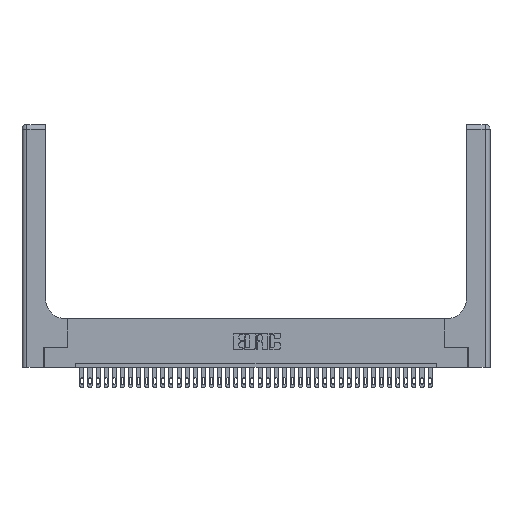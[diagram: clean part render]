
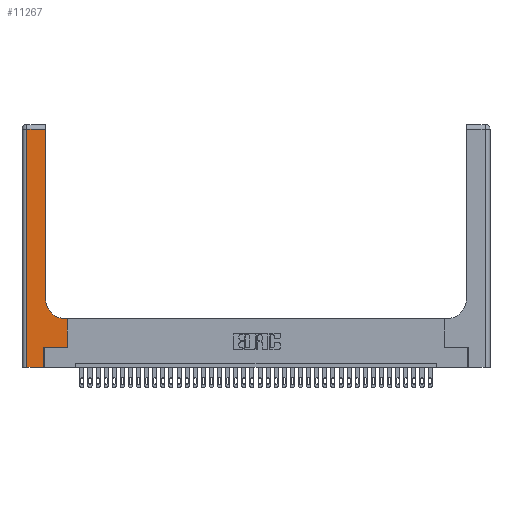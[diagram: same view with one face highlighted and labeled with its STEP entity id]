
A CAD part, top view. The second image highlights one B-rep face of the part: STEP entity #11267.
In plain terms, the highlighted planar face has unit normal (0, 0, 1).
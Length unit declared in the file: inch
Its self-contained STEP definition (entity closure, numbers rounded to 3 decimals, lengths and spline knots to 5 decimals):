
#680 = CARTESIAN_POINT ( 'NONE',  ( 0.06, 0., 0.37 ) ) ;
#816 = EDGE_CURVE ( 'NONE', #2927, #21546, #34071, .T. ) ;
#1588 = DIRECTION ( 'NONE',  ( 1., 0., 0. ) ) ;
#2129 = CARTESIAN_POINT ( 'NONE',  ( 0.2915, 3., 0.37 ) ) ;
#2460 = ORIENTED_EDGE ( 'NONE', *, *, #816, .T. ) ;
#2927 = VERTEX_POINT ( 'NONE', #27024 ) ;
#3459 = VECTOR ( 'NONE', #21099, 39.37008 ) ;
#3595 = ORIENTED_EDGE ( 'NONE', *, *, #24261, .T. ) ;
#3907 = CARTESIAN_POINT ( 'NONE',  ( 0.5585, 0.25, 0.37 ) ) ;
#4090 = ORIENTED_EDGE ( 'NONE', *, *, #33773, .T. ) ;
#4629 = VECTOR ( 'NONE', #26084, 39.37008 ) ;
#4866 = VERTEX_POINT ( 'NONE', #36740 ) ;
#4934 = DIRECTION ( 'NONE',  ( 1., 0., 0. ) ) ;
#5046 = EDGE_CURVE ( 'NONE', #28996, #8371, #12934, .T. ) ;
#5587 = DIRECTION ( 'NONE',  ( 0., 1., 0. ) ) ;
#5612 = PLANE ( 'NONE',  #34183 ) ;
#6397 = VECTOR ( 'NONE', #1588, 39.37008 ) ;
#6683 = EDGE_CURVE ( 'NONE', #35294, #28996, #28286, .T. ) ;
#8371 = VERTEX_POINT ( 'NONE', #13089 ) ;
#8490 = CARTESIAN_POINT ( 'NONE',  ( 0.5415, 0.6, 0.37 ) ) ;
#9694 = LINE ( 'NONE', #10641, #28366 ) ;
#9822 = ORIENTED_EDGE ( 'NONE', *, *, #26057, .T. ) ;
#10203 = VECTOR ( 'NONE', #5587, 39.37008 ) ;
#10488 = ORIENTED_EDGE ( 'NONE', *, *, #5046, .T. ) ;
#10577 = LINE ( 'NONE', #34936, #4629 ) ;
#10641 = CARTESIAN_POINT ( 'NONE',  ( 0.06, 3., 0.37 ) ) ;
#11267 = ADVANCED_FACE ( 'NONE', ( #24616 ), #5612, .F. ) ;
#11600 = ORIENTED_EDGE ( 'NONE', *, *, #12400, .T. ) ;
#11877 = ORIENTED_EDGE ( 'NONE', *, *, #37882, .T. ) ;
#11999 = CARTESIAN_POINT ( 'NONE',  ( 0.5585, 0.25, 0.37 ) ) ;
#12116 = CARTESIAN_POINT ( 'NONE',  ( 0.269, 0.25, 0.37 ) ) ;
#12400 = EDGE_CURVE ( 'NONE', #21546, #4866, #32258, .T. ) ;
#12431 = CIRCLE ( 'NONE', #13521, 0.25 ) ;
#12934 = LINE ( 'NONE', #3907, #10203 ) ;
#13089 = CARTESIAN_POINT ( 'NONE',  ( 0.5585, 0.6, 0.37 ) ) ;
#13521 = AXIS2_PLACEMENT_3D ( 'NONE', #31881, #22835, #16991 ) ;
#13764 = VECTOR ( 'NONE', #4934, 39.37008 ) ;
#16405 = CARTESIAN_POINT ( 'NONE',  ( 0.269, 0., 0.37 ) ) ;
#16991 = DIRECTION ( 'NONE',  ( 1., 0., 0. ) ) ;
#18083 = VERTEX_POINT ( 'NONE', #680 ) ;
#18611 = VERTEX_POINT ( 'NONE', #8490 ) ;
#19220 = DIRECTION ( 'NONE',  ( 0., -1., 0. ) ) ;
#19736 = ORIENTED_EDGE ( 'NONE', *, *, #6683, .T. ) ;
#20342 = EDGE_LOOP ( 'NONE', ( #2460, #11600, #11877, #23964, #3595, #19736, #10488, #9822, #4090 ) ) ;
#21099 = DIRECTION ( 'NONE',  ( -1., 0., 0. ) ) ;
#21546 = VERTEX_POINT ( 'NONE', #33022 ) ;
#22835 = DIRECTION ( 'NONE',  ( 0., 0., -1. ) ) ;
#23153 = DIRECTION ( 'NONE',  ( 0., 1., 0. ) ) ;
#23761 = VERTEX_POINT ( 'NONE', #26603 ) ;
#23964 = ORIENTED_EDGE ( 'NONE', *, *, #28215, .T. ) ;
#24261 = EDGE_CURVE ( 'NONE', #23761, #35294, #27606, .T. ) ;
#24437 = CARTESIAN_POINT ( 'NONE',  ( 0., 2.94, 0.37 ) ) ;
#24616 = FACE_OUTER_BOUND ( 'NONE', #20342, .T. ) ;
#26057 = EDGE_CURVE ( 'NONE', #8371, #18611, #10577, .T. ) ;
#26084 = DIRECTION ( 'NONE',  ( -1., 0., 0. ) ) ;
#26282 = DIRECTION ( 'NONE',  ( -1., 0., 0. ) ) ;
#26603 = CARTESIAN_POINT ( 'NONE',  ( 0.269, 0., 0.37 ) ) ;
#26694 = VECTOR ( 'NONE', #23153, 39.37008 ) ;
#27024 = CARTESIAN_POINT ( 'NONE',  ( 0.2915, 0.85, 0.37 ) ) ;
#27493 = CARTESIAN_POINT ( 'NONE',  ( 0.269, 0.25, 0.37 ) ) ;
#27606 = LINE ( 'NONE', #16405, #34972 ) ;
#28215 = EDGE_CURVE ( 'NONE', #18083, #23761, #31542, .T. ) ;
#28228 = DIRECTION ( 'NONE',  ( 0., 1., 0. ) ) ;
#28286 = LINE ( 'NONE', #27493, #6397 ) ;
#28366 = VECTOR ( 'NONE', #19220, 39.37008 ) ;
#28938 = CARTESIAN_POINT ( 'NONE',  ( 0., 3., 0.37 ) ) ;
#28996 = VERTEX_POINT ( 'NONE', #11999 ) ;
#31542 = LINE ( 'NONE', #37379, #13764 ) ;
#31881 = CARTESIAN_POINT ( 'NONE',  ( 0.5415, 0.85, 0.37 ) ) ;
#32258 = LINE ( 'NONE', #24437, #3459 ) ;
#33022 = CARTESIAN_POINT ( 'NONE',  ( 0.2915, 2.94, 0.37 ) ) ;
#33773 = EDGE_CURVE ( 'NONE', #18611, #2927, #12431, .T. ) ;
#34071 = LINE ( 'NONE', #2129, #26694 ) ;
#34183 = AXIS2_PLACEMENT_3D ( 'NONE', #28938, #35161, #26282 ) ;
#34936 = CARTESIAN_POINT ( 'NONE',  ( 0.2915, 0.6, 0.37 ) ) ;
#34972 = VECTOR ( 'NONE', #28228, 39.37008 ) ;
#35161 = DIRECTION ( 'NONE',  ( 0., 0., -1. ) ) ;
#35294 = VERTEX_POINT ( 'NONE', #12116 ) ;
#36740 = CARTESIAN_POINT ( 'NONE',  ( 0.06, 2.94, 0.37 ) ) ;
#37379 = CARTESIAN_POINT ( 'NONE',  ( 0., 0., 0.37 ) ) ;
#37882 = EDGE_CURVE ( 'NONE', #4866, #18083, #9694, .T. ) ;
